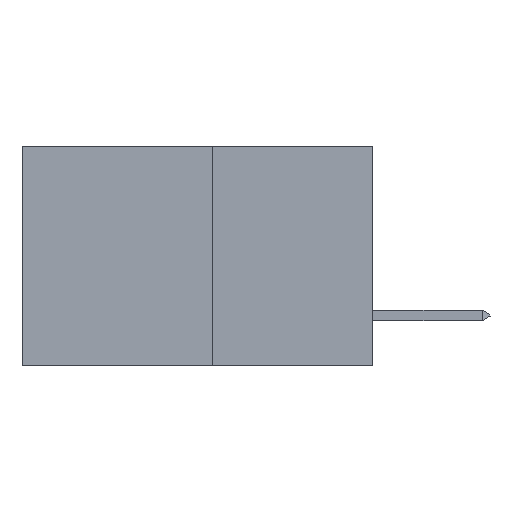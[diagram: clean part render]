
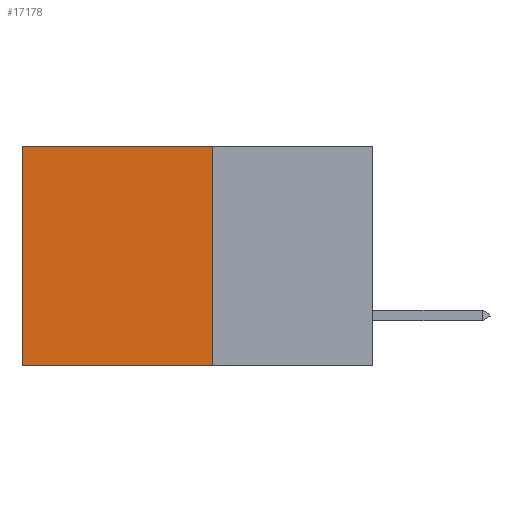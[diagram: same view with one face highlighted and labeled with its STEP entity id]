
A CAD part, left-side view. The second image highlights one B-rep face of the part: STEP entity #17178.
In plain terms, the highlighted planar face has unit normal (-1, 0, 0).
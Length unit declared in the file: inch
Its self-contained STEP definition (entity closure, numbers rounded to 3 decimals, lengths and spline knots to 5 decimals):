
#320 = AXIS2_PLACEMENT_3D ( 'NONE', #13523, #486, #29703 ) ;
#486 = DIRECTION ( 'NONE',  ( 1., 0., 0. ) ) ;
#1148 = CARTESIAN_POINT ( 'NONE',  ( 0.277, 0.27, -0.37 ) ) ;
#1540 = CARTESIAN_POINT ( 'NONE',  ( 0.277, 0.59, -0.37 ) ) ;
#2995 = VECTOR ( 'NONE', #13189, 39.37008 ) ;
#3298 = PLANE ( 'NONE',  #320 ) ;
#3754 = CARTESIAN_POINT ( 'NONE',  ( 0.277, 0.27, -0.37 ) ) ;
#4021 = ORIENTED_EDGE ( 'NONE', *, *, #25428, .T. ) ;
#4679 = EDGE_LOOP ( 'NONE', ( #4021, #18843, #21202, #11974 ) ) ;
#6041 = VECTOR ( 'NONE', #24188, 39.37008 ) ;
#6777 = LINE ( 'NONE', #12618, #6041 ) ;
#7423 = LINE ( 'NONE', #27028, #12898 ) ;
#8964 = EDGE_CURVE ( 'NONE', #25310, #29172, #27863, .T. ) ;
#10944 = DIRECTION ( 'NONE',  ( 0., 0., -1. ) ) ;
#11974 = ORIENTED_EDGE ( 'NONE', *, *, #28111, .T. ) ;
#12261 = CARTESIAN_POINT ( 'NONE',  ( 0.277, 0.59, -0.37 ) ) ;
#12618 = CARTESIAN_POINT ( 'NONE',  ( 0.277, 0.27, 0. ) ) ;
#12898 = VECTOR ( 'NONE', #10944, 39.37008 ) ;
#13189 = DIRECTION ( 'NONE',  ( 0., 0., -1. ) ) ;
#13523 = CARTESIAN_POINT ( 'NONE',  ( 0.277, 0.27, -0.37 ) ) ;
#16558 = VERTEX_POINT ( 'NONE', #28671 ) ;
#17178 = ADVANCED_FACE ( 'NONE', ( #22755 ), #3298, .F. ) ;
#17430 = DIRECTION ( 'NONE',  ( 0., 1., 0. ) ) ;
#18843 = ORIENTED_EDGE ( 'NONE', *, *, #8964, .F. ) ;
#18963 = EDGE_CURVE ( 'NONE', #16558, #25310, #7423, .T. ) ;
#21101 = VECTOR ( 'NONE', #17430, 39.37008 ) ;
#21202 = ORIENTED_EDGE ( 'NONE', *, *, #18963, .F. ) ;
#22679 = VERTEX_POINT ( 'NONE', #28590 ) ;
#22755 = FACE_OUTER_BOUND ( 'NONE', #4679, .T. ) ;
#24188 = DIRECTION ( 'NONE',  ( 0., 1., 0. ) ) ;
#25310 = VERTEX_POINT ( 'NONE', #1148 ) ;
#25428 = EDGE_CURVE ( 'NONE', #22679, #29172, #28229, .T. ) ;
#27028 = CARTESIAN_POINT ( 'NONE',  ( 0.277, 0.27, -0.37 ) ) ;
#27863 = LINE ( 'NONE', #3754, #21101 ) ;
#28111 = EDGE_CURVE ( 'NONE', #16558, #22679, #6777, .T. ) ;
#28229 = LINE ( 'NONE', #1540, #2995 ) ;
#28590 = CARTESIAN_POINT ( 'NONE',  ( 0.277, 0.59, 0. ) ) ;
#28671 = CARTESIAN_POINT ( 'NONE',  ( 0.277, 0.27, 0. ) ) ;
#29172 = VERTEX_POINT ( 'NONE', #12261 ) ;
#29703 = DIRECTION ( 'NONE',  ( 0., 0., -1. ) ) ;
